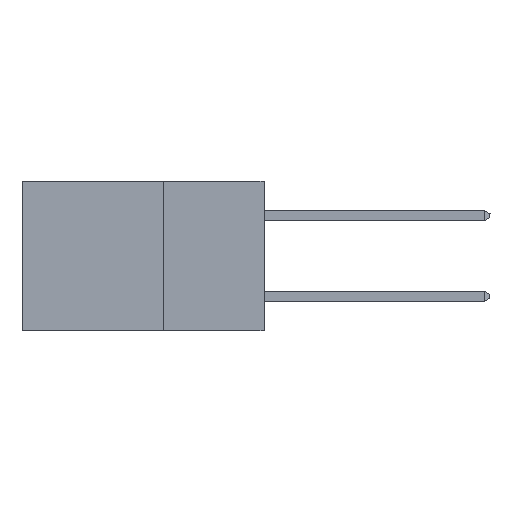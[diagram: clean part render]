
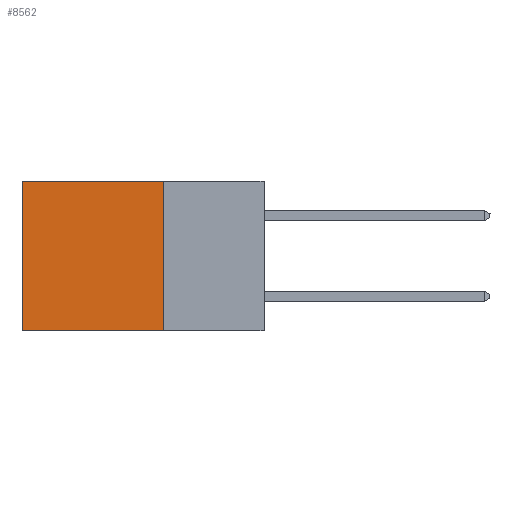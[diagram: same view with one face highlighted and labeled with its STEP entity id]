
A CAD part, left-side view. The second image highlights one B-rep face of the part: STEP entity #8562.
In plain terms, the highlighted planar face has unit normal (-1, 0, 0).
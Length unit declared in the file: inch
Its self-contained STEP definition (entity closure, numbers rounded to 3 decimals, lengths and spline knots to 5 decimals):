
#746 = LINE ( 'NONE', #20469, #21354 ) ;
#1004 = AXIS2_PLACEMENT_3D ( 'NONE', #21469, #9223, #23487 ) ;
#1270 = VERTEX_POINT ( 'NONE', #12112 ) ;
#1667 = EDGE_CURVE ( 'NONE', #3603, #10549, #7115, .T. ) ;
#3379 = ORIENTED_EDGE ( 'NONE', *, *, #18175, .T. ) ;
#3603 = VERTEX_POINT ( 'NONE', #23202 ) ;
#3996 = LINE ( 'NONE', #23251, #25113 ) ;
#4354 = VECTOR ( 'NONE', #5983, 39.37008 ) ;
#5983 = DIRECTION ( 'NONE',  ( 0., 0., -1. ) ) ;
#7115 = LINE ( 'NONE', #12280, #12524 ) ;
#8562 = ADVANCED_FACE ( 'NONE', ( #25841 ), #17391, .F. ) ;
#9223 = DIRECTION ( 'NONE',  ( 1., 0., 0. ) ) ;
#10116 = EDGE_CURVE ( 'NONE', #18227, #1270, #3996, .T. ) ;
#10269 = DIRECTION ( 'NONE',  ( 0., 0., -1. ) ) ;
#10549 = VERTEX_POINT ( 'NONE', #12262 ) ;
#12112 = CARTESIAN_POINT ( 'NONE',  ( 0.2615, 0.6, 0. ) ) ;
#12262 = CARTESIAN_POINT ( 'NONE',  ( 0.2615, 0.6, -0.37 ) ) ;
#12280 = CARTESIAN_POINT ( 'NONE',  ( 0.2615, 0.25, -0.37 ) ) ;
#12524 = VECTOR ( 'NONE', #14235, 39.37008 ) ;
#12906 = EDGE_LOOP ( 'NONE', ( #3379, #21071, #20428, #25566 ) ) ;
#14235 = DIRECTION ( 'NONE',  ( 0., 1., 0. ) ) ;
#14380 = CARTESIAN_POINT ( 'NONE',  ( 0.2615, 0.25, 0. ) ) ;
#15015 = EDGE_CURVE ( 'NONE', #18227, #3603, #20729, .T. ) ;
#17391 = PLANE ( 'NONE',  #1004 ) ;
#18175 = EDGE_CURVE ( 'NONE', #1270, #10549, #746, .T. ) ;
#18227 = VERTEX_POINT ( 'NONE', #14380 ) ;
#20428 = ORIENTED_EDGE ( 'NONE', *, *, #15015, .F. ) ;
#20469 = CARTESIAN_POINT ( 'NONE',  ( 0.2615, 0.6, -0.37 ) ) ;
#20729 = LINE ( 'NONE', #22324, #4354 ) ;
#21071 = ORIENTED_EDGE ( 'NONE', *, *, #1667, .F. ) ;
#21354 = VECTOR ( 'NONE', #10269, 39.37008 ) ;
#21469 = CARTESIAN_POINT ( 'NONE',  ( 0.2615, 0.25, -0.37 ) ) ;
#22324 = CARTESIAN_POINT ( 'NONE',  ( 0.2615, 0.25, -0.37 ) ) ;
#23202 = CARTESIAN_POINT ( 'NONE',  ( 0.2615, 0.25, -0.37 ) ) ;
#23251 = CARTESIAN_POINT ( 'NONE',  ( 0.2615, 0.25, 0. ) ) ;
#23487 = DIRECTION ( 'NONE',  ( 0., 0., -1. ) ) ;
#25113 = VECTOR ( 'NONE', #25289, 39.37008 ) ;
#25289 = DIRECTION ( 'NONE',  ( 0., 1., 0. ) ) ;
#25566 = ORIENTED_EDGE ( 'NONE', *, *, #10116, .T. ) ;
#25841 = FACE_OUTER_BOUND ( 'NONE', #12906, .T. ) ;
